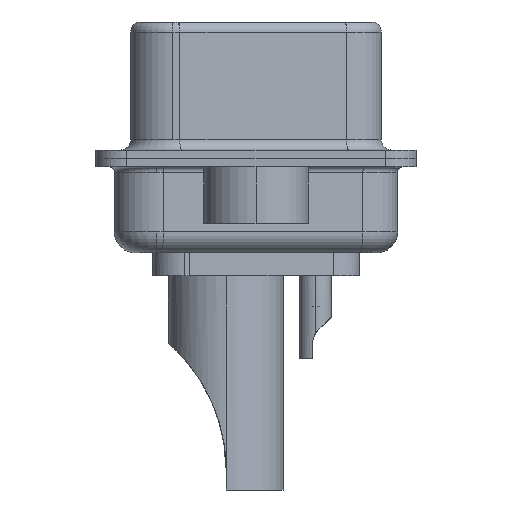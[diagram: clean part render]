
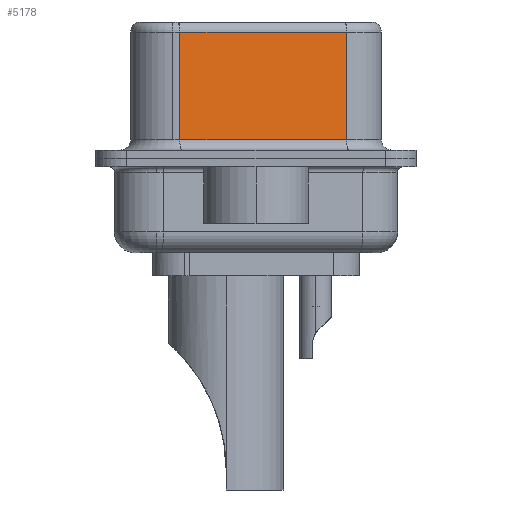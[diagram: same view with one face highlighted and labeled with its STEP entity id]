
A CAD part, left-side view. The second image highlights one B-rep face of the part: STEP entity #5178.
In plain terms, the highlighted planar face has unit normal (-0.985, -0.174, 0).
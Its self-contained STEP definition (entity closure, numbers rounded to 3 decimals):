
#511 = PLANE ( 'NONE',  #4140 ) ;
#1245 = VECTOR ( 'NONE', #4126, 1000. ) ;
#1502 = CARTESIAN_POINT ( 'NONE',  ( 5.132, -4.322, 6.02 ) ) ;
#1790 = VERTEX_POINT ( 'NONE', #24172 ) ;
#3391 = FACE_OUTER_BOUND ( 'NONE', #21426, .T. ) ;
#4126 = DIRECTION ( 'NONE',  ( 0., 0., -1. ) ) ;
#4140 = AXIS2_PLACEMENT_3D ( 'NONE', #20141, #26856, #26767 ) ;
#4332 = VECTOR ( 'NONE', #18972, 1000. ) ;
#4525 = VERTEX_POINT ( 'NONE', #1502 ) ;
#4661 = CARTESIAN_POINT ( 'NONE',  ( 5.132, -4.322, 0.9 ) ) ;
#4788 = ORIENTED_EDGE ( 'NONE', *, *, #20804, .T. ) ;
#5178 = ADVANCED_FACE ( 'NONE', ( #3391 ), #511, .F. ) ;
#7754 = DIRECTION ( 'NONE',  ( -0.174, 0.985, 0. ) ) ;
#8691 = CARTESIAN_POINT ( 'NONE',  ( 3.73, 3.628, 6.02 ) ) ;
#11802 = CARTESIAN_POINT ( 'NONE',  ( 5.132, -4.322, 6.02 ) ) ;
#14363 = CARTESIAN_POINT ( 'NONE',  ( 5.132, -4.322, 6.52 ) ) ;
#14705 = VECTOR ( 'NONE', #16489, 1000. ) ;
#14826 = ORIENTED_EDGE ( 'NONE', *, *, #25009, .T. ) ;
#15348 = LINE ( 'NONE', #18532, #14705 ) ;
#16448 = VECTOR ( 'NONE', #7754, 1000. ) ;
#16489 = DIRECTION ( 'NONE',  ( 0., 0., -1. ) ) ;
#16795 = VERTEX_POINT ( 'NONE', #8691 ) ;
#17295 = EDGE_CURVE ( 'NONE', #16795, #1790, #15348, .T. ) ;
#18532 = CARTESIAN_POINT ( 'NONE',  ( 3.73, 3.628, 6.52 ) ) ;
#18972 = DIRECTION ( 'NONE',  ( 0.174, -0.985, 0. ) ) ;
#19073 = CARTESIAN_POINT ( 'NONE',  ( 5.132, -4.322, 0.9 ) ) ;
#20141 = CARTESIAN_POINT ( 'NONE',  ( 5.132, -4.322, 6.52 ) ) ;
#20218 = EDGE_CURVE ( 'NONE', #4525, #24048, #23207, .T. ) ;
#20613 = LINE ( 'NONE', #4661, #4332 ) ;
#20804 = EDGE_CURVE ( 'NONE', #4525, #16795, #21858, .T. ) ;
#21426 = EDGE_LOOP ( 'NONE', ( #25488, #4788, #26514, #14826 ) ) ;
#21858 = LINE ( 'NONE', #11802, #16448 ) ;
#23207 = LINE ( 'NONE', #14363, #1245 ) ;
#24048 = VERTEX_POINT ( 'NONE', #19073 ) ;
#24172 = CARTESIAN_POINT ( 'NONE',  ( 3.73, 3.628, 0.9 ) ) ;
#25009 = EDGE_CURVE ( 'NONE', #1790, #24048, #20613, .T. ) ;
#25488 = ORIENTED_EDGE ( 'NONE', *, *, #20218, .F. ) ;
#26514 = ORIENTED_EDGE ( 'NONE', *, *, #17295, .T. ) ;
#26767 = DIRECTION ( 'NONE',  ( -0.174, 0.985, 0. ) ) ;
#26856 = DIRECTION ( 'NONE',  ( 0.985, 0.174, 0. ) ) ;
